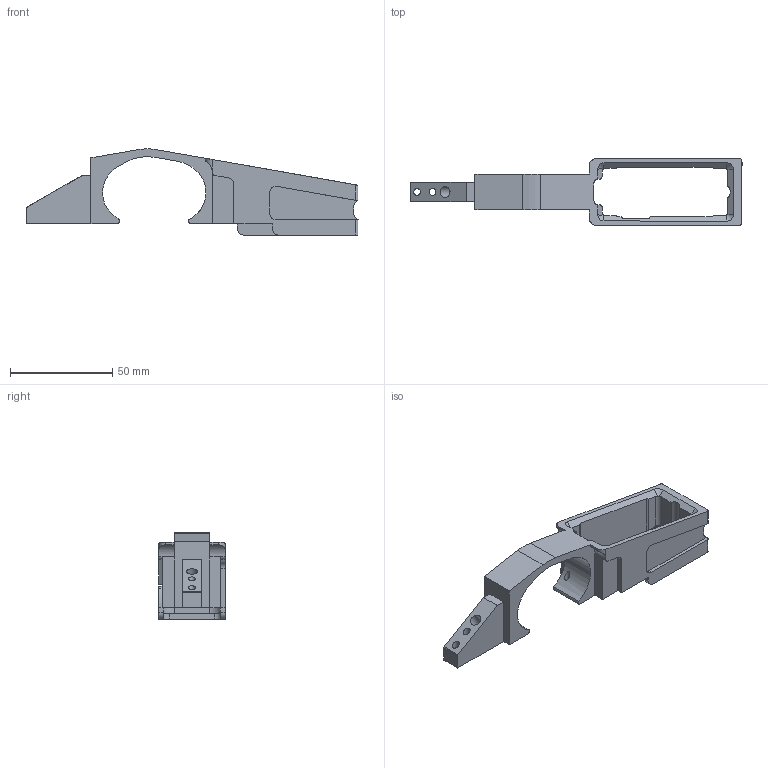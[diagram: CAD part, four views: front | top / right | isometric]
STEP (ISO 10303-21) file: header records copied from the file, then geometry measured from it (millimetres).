
FILE_DESCRIPTION(/* description */ (''),/* implementation_level */ '2;1');
FILE_NAME(/* name */ 'AR-00 Lower Lower v25.step',/* time_stamp */ '2022-01-13T16:26:55-06:00',/* author */ (''),/* organization */ (''),/* preprocessor_version */ 'ST-DEVELOPER v18.1',/* originating_system */ 'Autodesk Translation Framework v10.10.0.1391',/* authorisation */ '');
FILE_SCHEMA (('AUTOMOTIVE_DESIGN { 1 0 10303 214 3 1 1 }'));
Length unit declared in the file: inch
Products named in the file (1): AR-00 Lower Lower
Bounding box: 162.26 x 32.56 x 42.08 mm (x, y, z)
Volume: 32487 mm3; surface area: 19702.5 mm2
Topology: 1 solids, 1 shells, 126 faces, 365 edges, 239 vertices
Faces by surface type: plane 65, cylinder 57, cone 4
Full cylindrical faces by diameter (mm): 2.529 x1, 3.332 x2, 5.474 x1
Entity records: 4292 total; most frequent: CARTESIAN_POINT 813, DIRECTION 734, ORIENTED_EDGE 726, EDGE_CURVE 363, AXIS2_PLACEMENT_3D 250, VERTEX_POINT 239, LINE 234, VECTOR 234
